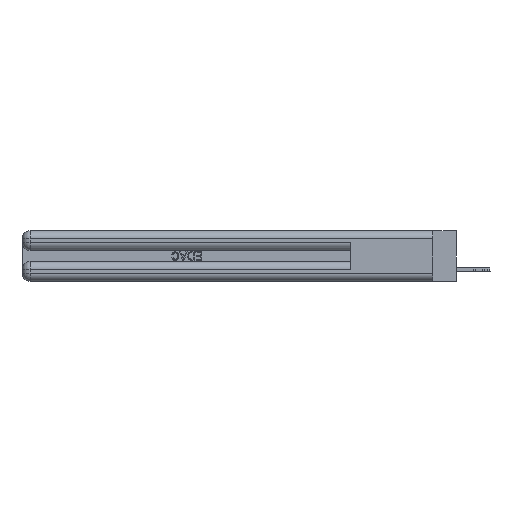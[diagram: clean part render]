
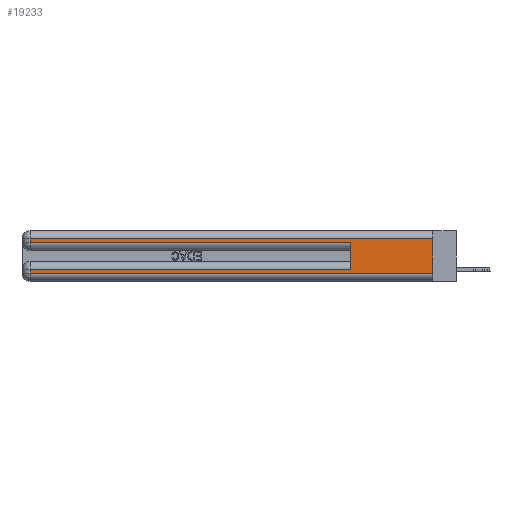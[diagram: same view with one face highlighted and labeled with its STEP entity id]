
A CAD part, left-side view. The second image highlights one B-rep face of the part: STEP entity #19233.
In plain terms, the highlighted planar face has unit normal (-1, 0, 0).
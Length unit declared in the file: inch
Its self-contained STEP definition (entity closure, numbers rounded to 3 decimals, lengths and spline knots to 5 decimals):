
#139 = FACE_OUTER_BOUND ( 'NONE', #7261, .T. ) ;
#251 = EDGE_CURVE ( 'NONE', #28598, #34242, #11253, .T. ) ;
#679 = ORIENTED_EDGE ( 'NONE', *, *, #17028, .T. ) ;
#1316 = ORIENTED_EDGE ( 'NONE', *, *, #37300, .F. ) ;
#2422 = VECTOR ( 'NONE', #11456, 39.37008 ) ;
#2856 = VERTEX_POINT ( 'NONE', #10132 ) ;
#3788 = LINE ( 'NONE', #27517, #37633 ) ;
#3848 = DIRECTION ( 'NONE',  ( 0., 0., -1. ) ) ;
#4719 = VECTOR ( 'NONE', #37400, 39.37008 ) ;
#4763 = CARTESIAN_POINT ( 'NONE',  ( 0., 2.94, 0.37 ) ) ;
#7261 = EDGE_LOOP ( 'NONE', ( #1316, #679, #16042, #16344, #31638, #42087, #10859, #24582 ) ) ;
#7889 = DIRECTION ( 'NONE',  ( 0., 0., -1. ) ) ;
#7910 = CARTESIAN_POINT ( 'NONE',  ( 0., 0.6, 0.285 ) ) ;
#8173 = VECTOR ( 'NONE', #32789, 39.37008 ) ;
#8184 = VECTOR ( 'NONE', #8884, 39.37008 ) ;
#8884 = DIRECTION ( 'NONE',  ( 0., -1., 0. ) ) ;
#9434 = VERTEX_POINT ( 'NONE', #24384 ) ;
#9891 = AXIS2_PLACEMENT_3D ( 'NONE', #29692, #20518, #7889 ) ;
#10097 = CARTESIAN_POINT ( 'NONE',  ( 0., 0., 0.37 ) ) ;
#10132 = CARTESIAN_POINT ( 'NONE',  ( 0., 2.94, 0.085 ) ) ;
#10319 = DIRECTION ( 'NONE',  ( 0., 0., 1. ) ) ;
#10322 = CARTESIAN_POINT ( 'NONE',  ( 0., 2.94, 0.37 ) ) ;
#10859 = ORIENTED_EDGE ( 'NONE', *, *, #35785, .T. ) ;
#10921 = LINE ( 'NONE', #10322, #12005 ) ;
#11253 = LINE ( 'NONE', #15438, #8184 ) ;
#11376 = LINE ( 'NONE', #13730, #16468 ) ;
#11456 = DIRECTION ( 'NONE',  ( 0., 1., 0. ) ) ;
#12005 = VECTOR ( 'NONE', #3848, 39.37008 ) ;
#13730 = CARTESIAN_POINT ( 'NONE',  ( 0., 0.6, 0.145 ) ) ;
#15438 = CARTESIAN_POINT ( 'NONE',  ( 0., 0., 0.285 ) ) ;
#16042 = ORIENTED_EDGE ( 'NONE', *, *, #17542, .T. ) ;
#16344 = ORIENTED_EDGE ( 'NONE', *, *, #251, .T. ) ;
#16468 = VECTOR ( 'NONE', #10319, 39.37008 ) ;
#17028 = EDGE_CURVE ( 'NONE', #24974, #30040, #3788, .T. ) ;
#17542 = EDGE_CURVE ( 'NONE', #30040, #28598, #10921, .T. ) ;
#19233 = ADVANCED_FACE ( 'NONE', ( #139 ), #30229, .F. ) ;
#20518 = DIRECTION ( 'NONE',  ( 1., 0., 0. ) ) ;
#23858 = VERTEX_POINT ( 'NONE', #25469 ) ;
#23885 = EDGE_CURVE ( 'NONE', #40116, #23858, #32057, .T. ) ;
#24384 = CARTESIAN_POINT ( 'NONE',  ( 0., 0.6, 0.085 ) ) ;
#24480 = LINE ( 'NONE', #10097, #8173 ) ;
#24582 = ORIENTED_EDGE ( 'NONE', *, *, #23885, .T. ) ;
#24974 = VERTEX_POINT ( 'NONE', #33937 ) ;
#25328 = CARTESIAN_POINT ( 'NONE',  ( 0., 0., 0.06 ) ) ;
#25469 = CARTESIAN_POINT ( 'NONE',  ( 0., 0., 0.06 ) ) ;
#25671 = CARTESIAN_POINT ( 'NONE',  ( 0., 2.94, 0.285 ) ) ;
#27517 = CARTESIAN_POINT ( 'NONE',  ( 0., 0., 0.31 ) ) ;
#28598 = VERTEX_POINT ( 'NONE', #25671 ) ;
#29692 = CARTESIAN_POINT ( 'NONE',  ( 0., 0., 0.37 ) ) ;
#29781 = CARTESIAN_POINT ( 'NONE',  ( 0., 2.94, 0.31 ) ) ;
#30040 = VERTEX_POINT ( 'NONE', #29781 ) ;
#30229 = PLANE ( 'NONE',  #9891 ) ;
#30790 = CARTESIAN_POINT ( 'NONE',  ( 0., 0., 0.085 ) ) ;
#30974 = VECTOR ( 'NONE', #34182, 39.37008 ) ;
#31638 = ORIENTED_EDGE ( 'NONE', *, *, #36132, .F. ) ;
#32057 = LINE ( 'NONE', #25328, #30974 ) ;
#32789 = DIRECTION ( 'NONE',  ( 0., 0., -1. ) ) ;
#33937 = CARTESIAN_POINT ( 'NONE',  ( 0., 0., 0.31 ) ) ;
#34182 = DIRECTION ( 'NONE',  ( 0., -1., 0. ) ) ;
#34242 = VERTEX_POINT ( 'NONE', #7910 ) ;
#34616 = LINE ( 'NONE', #30790, #2422 ) ;
#35785 = EDGE_CURVE ( 'NONE', #2856, #40116, #39569, .T. ) ;
#36132 = EDGE_CURVE ( 'NONE', #9434, #34242, #11376, .T. ) ;
#37300 = EDGE_CURVE ( 'NONE', #24974, #23858, #24480, .T. ) ;
#37400 = DIRECTION ( 'NONE',  ( 0., 0., -1. ) ) ;
#37483 = DIRECTION ( 'NONE',  ( 0., 1., 0. ) ) ;
#37633 = VECTOR ( 'NONE', #37483, 39.37008 ) ;
#39116 = EDGE_CURVE ( 'NONE', #9434, #2856, #34616, .T. ) ;
#39280 = CARTESIAN_POINT ( 'NONE',  ( 0., 2.94, 0.06 ) ) ;
#39569 = LINE ( 'NONE', #4763, #4719 ) ;
#40116 = VERTEX_POINT ( 'NONE', #39280 ) ;
#42087 = ORIENTED_EDGE ( 'NONE', *, *, #39116, .T. ) ;
